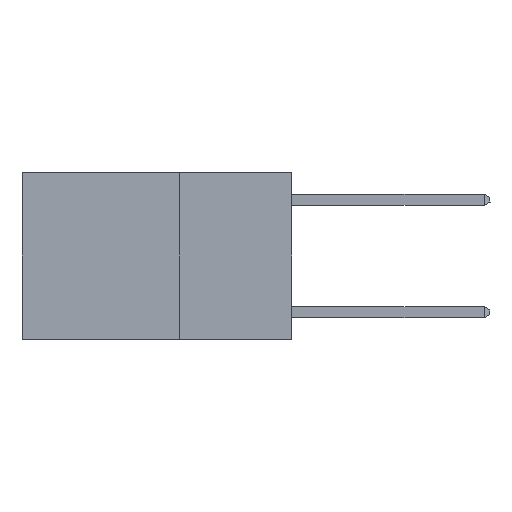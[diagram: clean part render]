
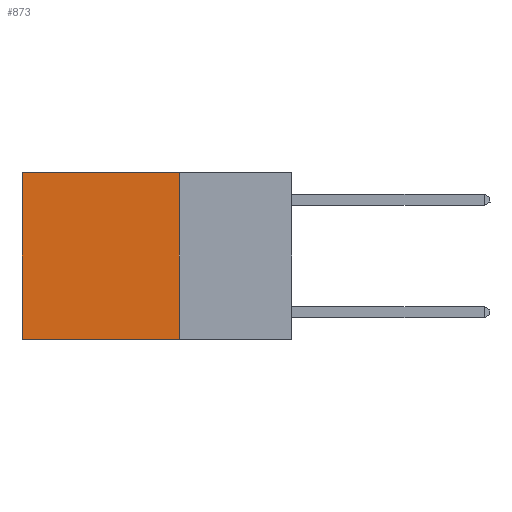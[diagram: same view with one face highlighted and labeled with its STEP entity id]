
A CAD part, left-side view. The second image highlights one B-rep face of the part: STEP entity #873.
In plain terms, the highlighted planar face has unit normal (-1, 0, 0).
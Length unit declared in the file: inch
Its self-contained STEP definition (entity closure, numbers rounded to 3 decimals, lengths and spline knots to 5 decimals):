
#256 = LINE ( 'NONE', #2252, #7734 ) ;
#832 = FACE_OUTER_BOUND ( 'NONE', #7470, .T. ) ;
#873 = ADVANCED_FACE ( 'NONE', ( #832 ), #9842, .F. ) ;
#1061 = DIRECTION ( 'NONE',  ( 0., 1., 0. ) ) ;
#1407 = CARTESIAN_POINT ( 'NONE',  ( 0.2625, 0.6, -0.37 ) ) ;
#2014 = CARTESIAN_POINT ( 'NONE',  ( 0.2625, 0.25, 0. ) ) ;
#2252 = CARTESIAN_POINT ( 'NONE',  ( 0.2625, 0.25, -0.37 ) ) ;
#2542 = VERTEX_POINT ( 'NONE', #11996 ) ;
#3045 = LINE ( 'NONE', #2014, #3624 ) ;
#3089 = ORIENTED_EDGE ( 'NONE', *, *, #3237, .F. ) ;
#3237 = EDGE_CURVE ( 'NONE', #11515, #9273, #3045, .T. ) ;
#3455 = AXIS2_PLACEMENT_3D ( 'NONE', #4177, #4090, #10820 ) ;
#3595 = ORIENTED_EDGE ( 'NONE', *, *, #7431, .F. ) ;
#3624 = VECTOR ( 'NONE', #6895, 39.37008 ) ;
#4000 = LINE ( 'NONE', #8740, #8843 ) ;
#4090 = DIRECTION ( 'NONE',  ( 1., 0., 0. ) ) ;
#4177 = CARTESIAN_POINT ( 'NONE',  ( 0.2625, 0.25, 0. ) ) ;
#4228 = VERTEX_POINT ( 'NONE', #1407 ) ;
#4891 = CARTESIAN_POINT ( 'NONE',  ( 0.2625, 0.25, -0.37 ) ) ;
#5142 = CARTESIAN_POINT ( 'NONE',  ( 0.2625, 0.25, 0. ) ) ;
#6014 = DIRECTION ( 'NONE',  ( 0., 0., -1. ) ) ;
#6315 = EDGE_CURVE ( 'NONE', #11515, #2542, #4000, .T. ) ;
#6424 = EDGE_CURVE ( 'NONE', #2542, #4228, #12000, .T. ) ;
#6895 = DIRECTION ( 'NONE',  ( 0., 0., -1. ) ) ;
#7371 = ORIENTED_EDGE ( 'NONE', *, *, #6424, .T. ) ;
#7431 = EDGE_CURVE ( 'NONE', #9273, #4228, #256, .T. ) ;
#7470 = EDGE_LOOP ( 'NONE', ( #7371, #3595, #3089, #8991 ) ) ;
#7734 = VECTOR ( 'NONE', #8892, 39.37008 ) ;
#8137 = CARTESIAN_POINT ( 'NONE',  ( 0.2625, 0.6, 0. ) ) ;
#8740 = CARTESIAN_POINT ( 'NONE',  ( 0.2625, 0.25, 0. ) ) ;
#8843 = VECTOR ( 'NONE', #1061, 39.37008 ) ;
#8892 = DIRECTION ( 'NONE',  ( 0., 1., 0. ) ) ;
#8991 = ORIENTED_EDGE ( 'NONE', *, *, #6315, .T. ) ;
#9273 = VERTEX_POINT ( 'NONE', #4891 ) ;
#9842 = PLANE ( 'NONE',  #3455 ) ;
#10300 = VECTOR ( 'NONE', #6014, 39.37008 ) ;
#10820 = DIRECTION ( 'NONE',  ( 0., 0., -1. ) ) ;
#11515 = VERTEX_POINT ( 'NONE', #5142 ) ;
#11996 = CARTESIAN_POINT ( 'NONE',  ( 0.2625, 0.6, 0. ) ) ;
#12000 = LINE ( 'NONE', #8137, #10300 ) ;
